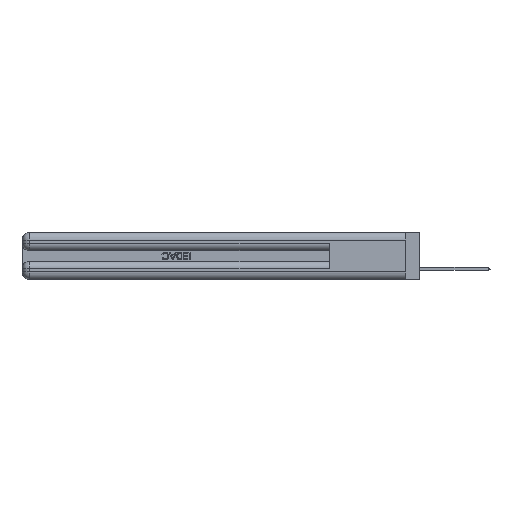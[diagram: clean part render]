
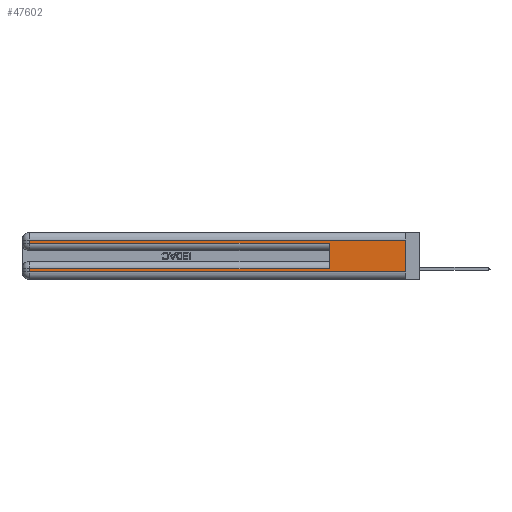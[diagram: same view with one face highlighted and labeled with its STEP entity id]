
A CAD part, left-side view. The second image highlights one B-rep face of the part: STEP entity #47602.
In plain terms, the highlighted planar face has unit normal (-1, 0, 0).
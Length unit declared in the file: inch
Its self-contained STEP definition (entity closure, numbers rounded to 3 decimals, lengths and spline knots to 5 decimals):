
#1219 = DIRECTION ( 'NONE',  ( 0., 0., -1. ) ) ;
#1299 = VECTOR ( 'NONE', #23750, 39.37008 ) ;
#1381 = DIRECTION ( 'NONE',  ( 0., -1., 0. ) ) ;
#2729 = LINE ( 'NONE', #11122, #34601 ) ;
#3108 = VECTOR ( 'NONE', #42794, 39.37008 ) ;
#3172 = ORIENTED_EDGE ( 'NONE', *, *, #38223, .T. ) ;
#4162 = FACE_OUTER_BOUND ( 'NONE', #22889, .T. ) ;
#5701 = VERTEX_POINT ( 'NONE', #13254 ) ;
#6436 = ORIENTED_EDGE ( 'NONE', *, *, #44684, .F. ) ;
#6594 = LINE ( 'NONE', #17636, #3108 ) ;
#6925 = CARTESIAN_POINT ( 'NONE',  ( 0., 0.6, 0.085 ) ) ;
#9378 = DIRECTION ( 'NONE',  ( 0., -1., 0. ) ) ;
#9828 = CARTESIAN_POINT ( 'NONE',  ( 0., 0., 0.37 ) ) ;
#10101 = ORIENTED_EDGE ( 'NONE', *, *, #42137, .T. ) ;
#10585 = EDGE_CURVE ( 'NONE', #23854, #37579, #6594, .T. ) ;
#11122 = CARTESIAN_POINT ( 'NONE',  ( 0., 2.94, 0.37 ) ) ;
#12274 = CARTESIAN_POINT ( 'NONE',  ( 0., 2.94, 0.37 ) ) ;
#13254 = CARTESIAN_POINT ( 'NONE',  ( 0., 0., 0.31 ) ) ;
#13775 = VECTOR ( 'NONE', #1381, 39.37008 ) ;
#14064 = CARTESIAN_POINT ( 'NONE',  ( 0., 0.6, 0.285 ) ) ;
#16125 = EDGE_CURVE ( 'NONE', #18730, #43689, #2729, .T. ) ;
#17091 = LINE ( 'NONE', #9828, #28732 ) ;
#17636 = CARTESIAN_POINT ( 'NONE',  ( 0., 0.6, 0.145 ) ) ;
#18730 = VERTEX_POINT ( 'NONE', #39883 ) ;
#19386 = CARTESIAN_POINT ( 'NONE',  ( 0., 2.94, 0.085 ) ) ;
#20153 = CARTESIAN_POINT ( 'NONE',  ( 0., 0., 0.06 ) ) ;
#20532 = ORIENTED_EDGE ( 'NONE', *, *, #10585, .F. ) ;
#20609 = DIRECTION ( 'NONE',  ( 0., 0., -1. ) ) ;
#21303 = CARTESIAN_POINT ( 'NONE',  ( 0., 0., 0.31 ) ) ;
#22889 = EDGE_LOOP ( 'NONE', ( #6436, #10101, #46078, #45000, #20532, #34994, #25737, #3172 ) ) ;
#23072 = VERTEX_POINT ( 'NONE', #35260 ) ;
#23750 = DIRECTION ( 'NONE',  ( 0., 0., -1. ) ) ;
#23854 = VERTEX_POINT ( 'NONE', #6925 ) ;
#25737 = ORIENTED_EDGE ( 'NONE', *, *, #29825, .T. ) ;
#25958 = LINE ( 'NONE', #47788, #13775 ) ;
#28732 = VECTOR ( 'NONE', #20609, 39.37008 ) ;
#29825 = EDGE_CURVE ( 'NONE', #46900, #23072, #35547, .T. ) ;
#30487 = VECTOR ( 'NONE', #9378, 39.37008 ) ;
#31381 = VECTOR ( 'NONE', #39817, 39.37008 ) ;
#32645 = CARTESIAN_POINT ( 'NONE',  ( 0., 0., 0.085 ) ) ;
#34601 = VECTOR ( 'NONE', #45925, 39.37008 ) ;
#34994 = ORIENTED_EDGE ( 'NONE', *, *, #47863, .T. ) ;
#35260 = CARTESIAN_POINT ( 'NONE',  ( 0., 2.94, 0.06 ) ) ;
#35547 = LINE ( 'NONE', #12274, #1299 ) ;
#36560 = VECTOR ( 'NONE', #47326, 39.37008 ) ;
#37132 = CARTESIAN_POINT ( 'NONE',  ( 0., 2.94, 0.285 ) ) ;
#37219 = LINE ( 'NONE', #32645, #31381 ) ;
#37579 = VERTEX_POINT ( 'NONE', #14064 ) ;
#38056 = EDGE_CURVE ( 'NONE', #43689, #37579, #25958, .T. ) ;
#38223 = EDGE_CURVE ( 'NONE', #23072, #43195, #42783, .T. ) ;
#38518 = CARTESIAN_POINT ( 'NONE',  ( 0., 0., 0.37 ) ) ;
#39817 = DIRECTION ( 'NONE',  ( 0., 1., 0. ) ) ;
#39883 = CARTESIAN_POINT ( 'NONE',  ( 0., 2.94, 0.31 ) ) ;
#42097 = DIRECTION ( 'NONE',  ( 1., 0., 0. ) ) ;
#42137 = EDGE_CURVE ( 'NONE', #5701, #18730, #46420, .T. ) ;
#42214 = CARTESIAN_POINT ( 'NONE',  ( 0., 0., 0.06 ) ) ;
#42783 = LINE ( 'NONE', #20153, #30487 ) ;
#42794 = DIRECTION ( 'NONE',  ( 0., 0., 1. ) ) ;
#43195 = VERTEX_POINT ( 'NONE', #42214 ) ;
#43689 = VERTEX_POINT ( 'NONE', #37132 ) ;
#44257 = AXIS2_PLACEMENT_3D ( 'NONE', #38518, #42097, #1219 ) ;
#44684 = EDGE_CURVE ( 'NONE', #5701, #43195, #17091, .T. ) ;
#45000 = ORIENTED_EDGE ( 'NONE', *, *, #38056, .T. ) ;
#45640 = PLANE ( 'NONE',  #44257 ) ;
#45925 = DIRECTION ( 'NONE',  ( 0., 0., -1. ) ) ;
#46078 = ORIENTED_EDGE ( 'NONE', *, *, #16125, .T. ) ;
#46420 = LINE ( 'NONE', #21303, #36560 ) ;
#46900 = VERTEX_POINT ( 'NONE', #19386 ) ;
#47326 = DIRECTION ( 'NONE',  ( 0., 1., 0. ) ) ;
#47602 = ADVANCED_FACE ( 'NONE', ( #4162 ), #45640, .F. ) ;
#47788 = CARTESIAN_POINT ( 'NONE',  ( 0., 0., 0.285 ) ) ;
#47863 = EDGE_CURVE ( 'NONE', #23854, #46900, #37219, .T. ) ;
